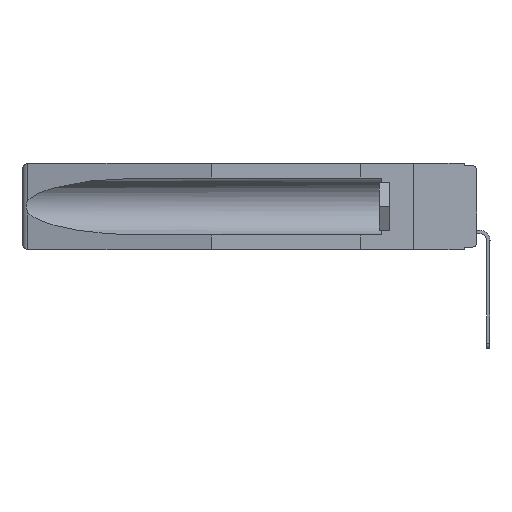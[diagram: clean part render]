
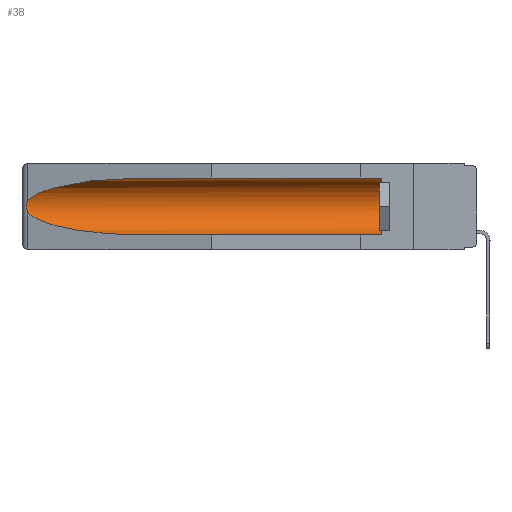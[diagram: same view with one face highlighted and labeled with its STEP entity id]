
A CAD part, left-side view. The second image highlights one B-rep face of the part: STEP entity #38.
In plain terms, the highlighted cylindrical face has radius 2.857 mm (diameter 5.715 mm), a partial arc.
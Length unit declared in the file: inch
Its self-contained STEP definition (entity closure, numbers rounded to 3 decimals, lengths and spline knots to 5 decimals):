
#38 = ADVANCED_FACE ( 'NONE', ( #9358 ), #13323, .F. ) ;
#99 = EDGE_CURVE ( 'NONE', #22737, #3018, #9221, .T. ) ;
#960 = CARTESIAN_POINT ( 'NONE',  ( 0.26537, 1.52718, -0.14972 ) ) ;
#1096 = CARTESIAN_POINT ( 'NONE',  ( 0.26655, 1.53094, -0.18657 ) ) ;
#1649 = DIRECTION ( 'NONE',  ( 0., 1., 0. ) ) ;
#2376 = CARTESIAN_POINT ( 'NONE',  ( 0.155, 0.126, -0.059 ) ) ;
#2583 = CARTESIAN_POINT ( 'NONE',  ( 0.26537, 1.52718, -0.19328 ) ) ;
#3018 = VERTEX_POINT ( 'NONE', #12280 ) ;
#3057 = CARTESIAN_POINT ( 'NONE',  ( 0.26654, 1.53092, -0.15636 ) ) ;
#4346 = EDGE_CURVE ( 'NONE', #11352, #15584, #10584, .T. ) ;
#4397 = VECTOR ( 'NONE', #8352, 39.37008 ) ;
#5412 = DIRECTION ( 'NONE',  ( 0., 0., 1. ) ) ;
#5660 = CARTESIAN_POINT ( 'NONE',  ( 0.155, 1.07973, -0.284 ) ) ;
#5958 = DIRECTION ( 'NONE',  ( 0., 0., 1. ) ) ;
#6195 = AXIS2_PLACEMENT_3D ( 'NONE', #19304, #23527, #5412 ) ;
#6629 = LINE ( 'NONE', #22387, #4397 ) ;
#8091 = EDGE_CURVE ( 'NONE', #11352, #3018, #6629, .T. ) ;
#8352 = DIRECTION ( 'NONE',  ( 0., 1., 0. ) ) ;
#9221 =( BOUNDED_CURVE ( )  B_SPLINE_CURVE ( 3, ( #21030, #13848, #26017, #5660 ),
 .UNSPECIFIED., .F., .F. ) 
 B_SPLINE_CURVE_WITH_KNOTS ( ( 4, 4 ),
 ( 0.1948, 1.5708 ),
 .UNSPECIFIED. ) 
 CURVE ( )  GEOMETRIC_REPRESENTATION_ITEM ( )  RATIONAL_B_SPLINE_CURVE ( ( 1., 0.848, 0.848, 1. ) ) 
 REPRESENTATION_ITEM ( '' )  );
#9267 = CARTESIAN_POINT ( 'NONE',  ( 0.2673, 1.53269, -0.17917 ) ) ;
#9358 = FACE_OUTER_BOUND ( 'NONE', #9611, .T. ) ;
#9611 = EDGE_LOOP ( 'NONE', ( #15774, #26092, #10843, #16773, #24692, #13891 ) ) ;
#10584 = CIRCLE ( 'NONE', #25381, 0.1125 ) ;
#10843 = ORIENTED_EDGE ( 'NONE', *, *, #99, .T. ) ;
#10965 = CARTESIAN_POINT ( 'NONE',  ( 0.26537, 1.52718, -0.19328 ) ) ;
#11231 = CARTESIAN_POINT ( 'NONE',  ( 0.2675, 1.53308, -0.17534 ) ) ;
#11352 = VERTEX_POINT ( 'NONE', #18712 ) ;
#11613 = VERTEX_POINT ( 'NONE', #20013 ) ;
#11661 = CARTESIAN_POINT ( 'NONE',  ( 0.155, -0.30754, -0.059 ) ) ;
#12280 = CARTESIAN_POINT ( 'NONE',  ( 0.155, 1.07973, -0.284 ) ) ;
#12963 = CARTESIAN_POINT ( 'NONE',  ( 0.26597, 1.5296, -0.19026 ) ) ;
#13215 = CARTESIAN_POINT ( 'NONE',  ( 0.2675, 1.53308, -0.16763 ) ) ;
#13323 = CYLINDRICAL_SURFACE ( 'NONE', #6195, 0.1125 ) ;
#13848 = CARTESIAN_POINT ( 'NONE',  ( 0.25451, 1.48313, -0.24835 ) ) ;
#13891 = ORIENTED_EDGE ( 'NONE', *, *, #25933, .T. ) ;
#14749 = VECTOR ( 'NONE', #1649, 39.37008 ) ;
#15584 = VERTEX_POINT ( 'NONE', #2376 ) ;
#15755 = CARTESIAN_POINT ( 'NONE',  ( 0.25451, 1.48313, -0.09465 ) ) ;
#15774 = ORIENTED_EDGE ( 'NONE', *, *, #17613, .T. ) ;
#16773 = ORIENTED_EDGE ( 'NONE', *, *, #8091, .F. ) ;
#17242 = CARTESIAN_POINT ( 'NONE',  ( 0.155, 1.07973, -0.059 ) ) ;
#17507 = LINE ( 'NONE', #11661, #14749 ) ;
#17549 = B_SPLINE_CURVE_WITH_KNOTS ( 'NONE', 3,
 ( #960, #21578, #3057, #23290, #13215, #11231, #9267, #1096, #12963, #10965 ),
 .UNSPECIFIED., .F., .F.,
 ( 4, 2, 2, 2, 4 ),
 ( 0., 0.00029, 0.00058, 0.00087, 0.00117 ),
 .UNSPECIFIED. ) ;
#17613 = EDGE_CURVE ( 'NONE', #11613, #22947, #21055, .T. ) ;
#17773 = CARTESIAN_POINT ( 'NONE',  ( 0.21114, 1.30732, -0.059 ) ) ;
#18712 = CARTESIAN_POINT ( 'NONE',  ( 0.155, 0.126, -0.284 ) ) ;
#19304 = CARTESIAN_POINT ( 'NONE',  ( 0.155, -0.30754, -0.1715 ) ) ;
#19634 = CARTESIAN_POINT ( 'NONE',  ( 0.26537, 1.52718, -0.14972 ) ) ;
#20013 = CARTESIAN_POINT ( 'NONE',  ( 0.155, 1.07973, -0.059 ) ) ;
#21030 = CARTESIAN_POINT ( 'NONE',  ( 0.26537, 1.52718, -0.19328 ) ) ;
#21055 =( BOUNDED_CURVE ( )  B_SPLINE_CURVE ( 3, ( #17242, #17773, #15755, #19634 ),
 .UNSPECIFIED., .F., .F. ) 
 B_SPLINE_CURVE_WITH_KNOTS ( ( 4, 4 ),
 ( 4.71239, 6.08839 ),
 .UNSPECIFIED. ) 
 CURVE ( )  GEOMETRIC_REPRESENTATION_ITEM ( )  RATIONAL_B_SPLINE_CURVE ( ( 1., 0.848, 0.848, 1. ) ) 
 REPRESENTATION_ITEM ( '' )  );
#21578 = CARTESIAN_POINT ( 'NONE',  ( 0.26597, 1.52961, -0.15275 ) ) ;
#21644 = EDGE_CURVE ( 'NONE', #22947, #22737, #17549, .T. ) ;
#21974 = DIRECTION ( 'NONE',  ( 0., -1., 0. ) ) ;
#22387 = CARTESIAN_POINT ( 'NONE',  ( 0.155, -0.30754, -0.284 ) ) ;
#22737 = VERTEX_POINT ( 'NONE', #2583 ) ;
#22947 = VERTEX_POINT ( 'NONE', #25693 ) ;
#23290 = CARTESIAN_POINT ( 'NONE',  ( 0.2673, 1.5327, -0.16383 ) ) ;
#23527 = DIRECTION ( 'NONE',  ( 0., 1., 0. ) ) ;
#24692 = ORIENTED_EDGE ( 'NONE', *, *, #4346, .T. ) ;
#25381 = AXIS2_PLACEMENT_3D ( 'NONE', #25908, #21974, #5958 ) ;
#25693 = CARTESIAN_POINT ( 'NONE',  ( 0.26537, 1.52718, -0.14972 ) ) ;
#25908 = CARTESIAN_POINT ( 'NONE',  ( 0.155, 0.126, -0.1715 ) ) ;
#25933 = EDGE_CURVE ( 'NONE', #15584, #11613, #17507, .T. ) ;
#26017 = CARTESIAN_POINT ( 'NONE',  ( 0.21114, 1.30732, -0.284 ) ) ;
#26092 = ORIENTED_EDGE ( 'NONE', *, *, #21644, .T. ) ;
